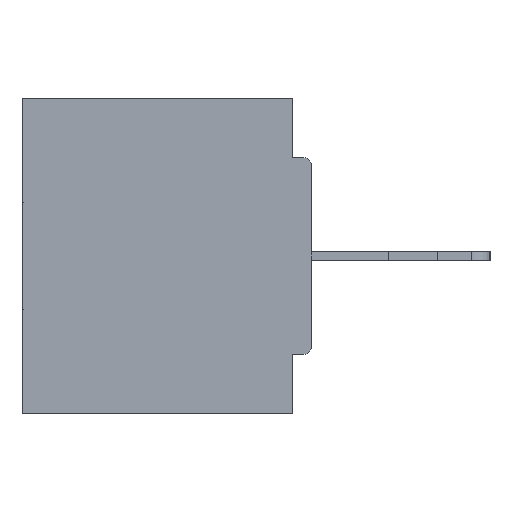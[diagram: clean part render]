
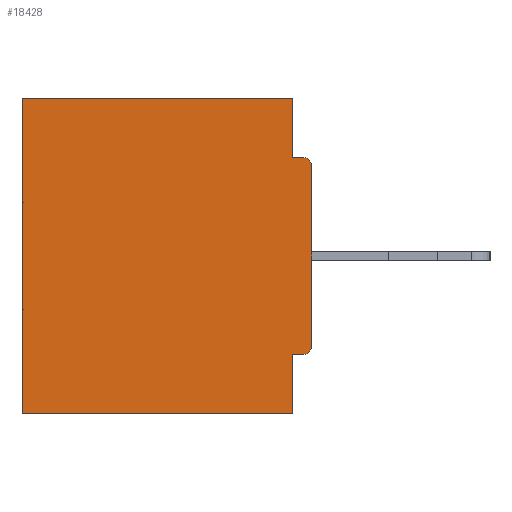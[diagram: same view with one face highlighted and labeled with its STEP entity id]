
A CAD part, left-side view. The second image highlights one B-rep face of the part: STEP entity #18428.
In plain terms, the highlighted planar face has unit normal (-1, 0, 0).
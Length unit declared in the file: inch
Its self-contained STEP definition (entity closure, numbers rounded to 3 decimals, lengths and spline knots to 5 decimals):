
#48 = AXIS2_PLACEMENT_3D ( 'NONE', #32529, #27274, #16353 ) ;
#96 = DIRECTION ( 'NONE',  ( 0., 0., -1. ) ) ;
#238 = VECTOR ( 'NONE', #6897, 39.37008 ) ;
#1327 = CARTESIAN_POINT ( 'NONE',  ( 0.298, 0.031, -0.5 ) ) ;
#1590 = ORIENTED_EDGE ( 'NONE', *, *, #4931, .T. ) ;
#1868 = VECTOR ( 'NONE', #15433, 39.37008 ) ;
#2871 = DIRECTION ( 'NONE',  ( 0., 0., -1. ) ) ;
#2975 = EDGE_CURVE ( 'NONE', #27048, #35701, #29460, .T. ) ;
#3189 = DIRECTION ( 'NONE',  ( 1., 0., 0. ) ) ;
#3268 = CARTESIAN_POINT ( 'NONE',  ( 0.298, 0.46, -0.5 ) ) ;
#3439 = VERTEX_POINT ( 'NONE', #6936 ) ;
#4325 = VECTOR ( 'NONE', #2871, 39.37008 ) ;
#4391 = CARTESIAN_POINT ( 'NONE',  ( 0.298, 0.031, -0.5 ) ) ;
#4766 = DIRECTION ( 'NONE',  ( -1., 0., 0. ) ) ;
#4931 = EDGE_CURVE ( 'NONE', #3439, #27048, #27483, .T. ) ;
#5256 = CARTESIAN_POINT ( 'NONE',  ( 0.298, 0., -0.3915 ) ) ;
#5543 = ORIENTED_EDGE ( 'NONE', *, *, #5710, .F. ) ;
#5690 = ORIENTED_EDGE ( 'NONE', *, *, #9702, .T. ) ;
#5710 = EDGE_CURVE ( 'NONE', #34878, #27405, #19173, .T. ) ;
#5963 = LINE ( 'NONE', #6150, #33733 ) ;
#6062 = AXIS2_PLACEMENT_3D ( 'NONE', #31104, #3189, #17675 ) ;
#6150 = CARTESIAN_POINT ( 'NONE',  ( 0.298, 0., -0.4065 ) ) ;
#6657 = AXIS2_PLACEMENT_3D ( 'NONE', #24180, #4766, #27448 ) ;
#6897 = DIRECTION ( 'NONE',  ( 0., 1., 0. ) ) ;
#6936 = CARTESIAN_POINT ( 'NONE',  ( 0.298, 0.031, 0. ) ) ;
#7698 = DIRECTION ( 'NONE',  ( 0., 0., -1. ) ) ;
#9347 = PLANE ( 'NONE',  #6062 ) ;
#9511 = EDGE_LOOP ( 'NONE', ( #5690, #23299, #18466, #1590, #25874, #32544, #26663, #21314, #18588, #5543 ) ) ;
#9702 = EDGE_CURVE ( 'NONE', #34878, #14146, #19114, .T. ) ;
#10308 = CARTESIAN_POINT ( 'NONE',  ( 0.298, 0., -0.5 ) ) ;
#10363 = CARTESIAN_POINT ( 'NONE',  ( 0.298, 0.46, 0. ) ) ;
#10521 = VERTEX_POINT ( 'NONE', #32272 ) ;
#11296 = EDGE_CURVE ( 'NONE', #33568, #19949, #29250, .T. ) ;
#11605 = DIRECTION ( 'NONE',  ( 0., -1., 0. ) ) ;
#11625 = CARTESIAN_POINT ( 'NONE',  ( 0.298, 0., 0. ) ) ;
#12818 = CARTESIAN_POINT ( 'NONE',  ( 0.298, 0.031, -0.5 ) ) ;
#12867 = EDGE_CURVE ( 'NONE', #19949, #35701, #18097, .T. ) ;
#14146 = VERTEX_POINT ( 'NONE', #29921 ) ;
#15262 = VECTOR ( 'NONE', #26765, 39.37008 ) ;
#15433 = DIRECTION ( 'NONE',  ( 0., 0., -1. ) ) ;
#16353 = DIRECTION ( 'NONE',  ( 0., 0., -1. ) ) ;
#16529 = LINE ( 'NONE', #19577, #35069 ) ;
#17675 = DIRECTION ( 'NONE',  ( 0., 0., -1. ) ) ;
#18097 = LINE ( 'NONE', #10308, #238 ) ;
#18428 = ADVANCED_FACE ( 'NONE', ( #25700 ), #9347, .F. ) ;
#18466 = ORIENTED_EDGE ( 'NONE', *, *, #27860, .F. ) ;
#18588 = ORIENTED_EDGE ( 'NONE', *, *, #29584, .T. ) ;
#19114 = CIRCLE ( 'NONE', #48, 0.015 ) ;
#19173 = LINE ( 'NONE', #11625, #4325 ) ;
#19577 = CARTESIAN_POINT ( 'NONE',  ( 0.298, 0., -0.0935 ) ) ;
#19949 = VERTEX_POINT ( 'NONE', #1327 ) ;
#19950 = VECTOR ( 'NONE', #96, 39.37008 ) ;
#21314 = ORIENTED_EDGE ( 'NONE', *, *, #24697, .F. ) ;
#22266 = CIRCLE ( 'NONE', #6657, 0.015 ) ;
#22622 = DIRECTION ( 'NONE',  ( 0., 1., 0. ) ) ;
#23284 = CARTESIAN_POINT ( 'NONE',  ( 0.298, 0.031, -0.4065 ) ) ;
#23299 = ORIENTED_EDGE ( 'NONE', *, *, #29664, .F. ) ;
#24180 = CARTESIAN_POINT ( 'NONE',  ( 0.298, 0.015, -0.3915 ) ) ;
#24697 = EDGE_CURVE ( 'NONE', #25329, #33568, #5963, .T. ) ;
#25329 = VERTEX_POINT ( 'NONE', #27298 ) ;
#25700 = FACE_OUTER_BOUND ( 'NONE', #9511, .T. ) ;
#25874 = ORIENTED_EDGE ( 'NONE', *, *, #2975, .T. ) ;
#26663 = ORIENTED_EDGE ( 'NONE', *, *, #11296, .F. ) ;
#26765 = DIRECTION ( 'NONE',  ( 0., 1., 0. ) ) ;
#27048 = VERTEX_POINT ( 'NONE', #10363 ) ;
#27274 = DIRECTION ( 'NONE',  ( -1., 0., 0. ) ) ;
#27298 = CARTESIAN_POINT ( 'NONE',  ( 0.298, 0.015, -0.4065 ) ) ;
#27405 = VERTEX_POINT ( 'NONE', #5256 ) ;
#27448 = DIRECTION ( 'NONE',  ( 0., 0., -1. ) ) ;
#27483 = LINE ( 'NONE', #29468, #15262 ) ;
#27860 = EDGE_CURVE ( 'NONE', #3439, #10521, #30192, .T. ) ;
#29250 = LINE ( 'NONE', #4391, #1868 ) ;
#29460 = LINE ( 'NONE', #34913, #29634 ) ;
#29468 = CARTESIAN_POINT ( 'NONE',  ( 0.298, 0., 0. ) ) ;
#29584 = EDGE_CURVE ( 'NONE', #25329, #27405, #22266, .T. ) ;
#29634 = VECTOR ( 'NONE', #7698, 39.37008 ) ;
#29664 = EDGE_CURVE ( 'NONE', #10521, #14146, #16529, .T. ) ;
#29921 = CARTESIAN_POINT ( 'NONE',  ( 0.298, 0.015, -0.0935 ) ) ;
#30192 = LINE ( 'NONE', #12818, #19950 ) ;
#31104 = CARTESIAN_POINT ( 'NONE',  ( 0.298, 0., 0. ) ) ;
#31649 = CARTESIAN_POINT ( 'NONE',  ( 0.298, 0., -0.1085 ) ) ;
#32272 = CARTESIAN_POINT ( 'NONE',  ( 0.298, 0.031, -0.0935 ) ) ;
#32529 = CARTESIAN_POINT ( 'NONE',  ( 0.298, 0.015, -0.1085 ) ) ;
#32544 = ORIENTED_EDGE ( 'NONE', *, *, #12867, .F. ) ;
#33568 = VERTEX_POINT ( 'NONE', #23284 ) ;
#33733 = VECTOR ( 'NONE', #22622, 39.37008 ) ;
#34878 = VERTEX_POINT ( 'NONE', #31649 ) ;
#34913 = CARTESIAN_POINT ( 'NONE',  ( 0.298, 0.46, 0. ) ) ;
#35069 = VECTOR ( 'NONE', #11605, 39.37008 ) ;
#35701 = VERTEX_POINT ( 'NONE', #3268 ) ;
